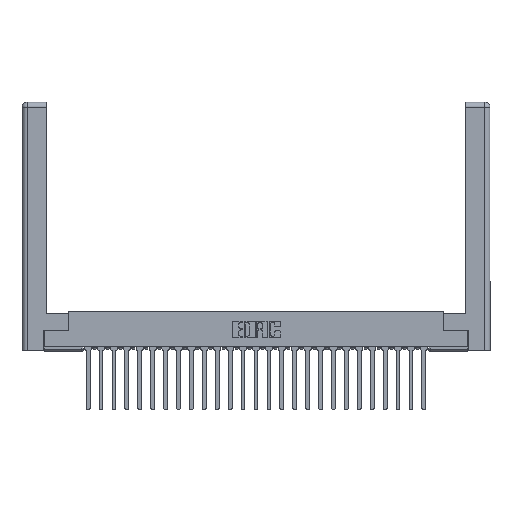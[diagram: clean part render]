
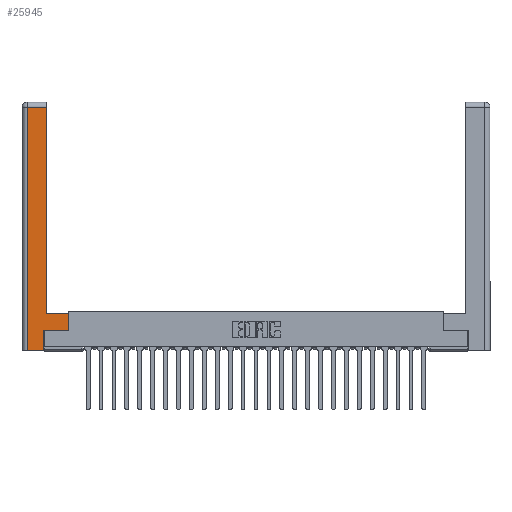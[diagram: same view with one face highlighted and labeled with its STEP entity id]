
A CAD part, top view. The second image highlights one B-rep face of the part: STEP entity #25945.
In plain terms, the highlighted planar face has unit normal (0, 0, 1).
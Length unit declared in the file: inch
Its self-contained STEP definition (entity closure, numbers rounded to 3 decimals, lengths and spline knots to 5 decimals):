
#501 = VECTOR ( 'NONE', #23197, 39.37008 ) ;
#703 = CARTESIAN_POINT ( 'NONE',  ( 0.265, 0., 0. ) ) ;
#752 = CARTESIAN_POINT ( 'NONE',  ( 0.295, 3., 0. ) ) ;
#923 = EDGE_CURVE ( 'NONE', #23110, #20462, #10369, .T. ) ;
#1741 = CARTESIAN_POINT ( 'NONE',  ( 0.265, 0., 0. ) ) ;
#1751 = CARTESIAN_POINT ( 'NONE',  ( 0.0615, 0., 0. ) ) ;
#2740 = LINE ( 'NONE', #17541, #24730 ) ;
#3184 = VECTOR ( 'NONE', #8556, 39.37008 ) ;
#4486 = ORIENTED_EDGE ( 'NONE', *, *, #923, .T. ) ;
#5169 = EDGE_CURVE ( 'NONE', #17542, #25307, #2740, .T. ) ;
#5480 = ORIENTED_EDGE ( 'NONE', *, *, #22704, .T. ) ;
#6525 = LINE ( 'NONE', #6589, #3184 ) ;
#6589 = CARTESIAN_POINT ( 'NONE',  ( 0.565, 0.245, 0. ) ) ;
#6923 = DIRECTION ( 'NONE',  ( 0., 1., 0. ) ) ;
#7065 = CARTESIAN_POINT ( 'NONE',  ( 0.0615, 2.94, 0. ) ) ;
#7544 = VECTOR ( 'NONE', #14274, 39.37008 ) ;
#8556 = DIRECTION ( 'NONE',  ( 1., 0., 0. ) ) ;
#9520 = EDGE_LOOP ( 'NONE', ( #11846, #4486, #5480, #23843, #16336, #23941, #27568, #16644 ) ) ;
#9521 = CARTESIAN_POINT ( 'NONE',  ( 0.295, 2.94, 0. ) ) ;
#9962 = LINE ( 'NONE', #27086, #10650 ) ;
#10175 = DIRECTION ( 'NONE',  ( 0., 0., -1. ) ) ;
#10263 = DIRECTION ( 'NONE',  ( -1., 0., 0. ) ) ;
#10369 = LINE ( 'NONE', #23160, #19050 ) ;
#10650 = VECTOR ( 'NONE', #18647, 39.37008 ) ;
#11282 = VERTEX_POINT ( 'NONE', #23946 ) ;
#11846 = ORIENTED_EDGE ( 'NONE', *, *, #24681, .T. ) ;
#12591 = DIRECTION ( 'NONE',  ( -1., 0., 0. ) ) ;
#13176 = EDGE_CURVE ( 'NONE', #16482, #17907, #6525, .T. ) ;
#14007 = EDGE_CURVE ( 'NONE', #11282, #20609, #21494, .T. ) ;
#14274 = DIRECTION ( 'NONE',  ( 0., 1., 0. ) ) ;
#16336 = ORIENTED_EDGE ( 'NONE', *, *, #25843, .T. ) ;
#16482 = VERTEX_POINT ( 'NONE', #22584 ) ;
#16644 = ORIENTED_EDGE ( 'NONE', *, *, #5169, .T. ) ;
#16682 = PLANE ( 'NONE',  #26206 ) ;
#16854 = LINE ( 'NONE', #1751, #501 ) ;
#16864 = CARTESIAN_POINT ( 'NONE',  ( 0., 0., 0. ) ) ;
#17541 = CARTESIAN_POINT ( 'NONE',  ( 0.295, 0.45, 0. ) ) ;
#17542 = VERTEX_POINT ( 'NONE', #21168 ) ;
#17543 = LINE ( 'NONE', #18364, #7544 ) ;
#17907 = VERTEX_POINT ( 'NONE', #20570 ) ;
#18364 = CARTESIAN_POINT ( 'NONE',  ( 0.265, 0.245, 0. ) ) ;
#18647 = DIRECTION ( 'NONE',  ( 0., 1., 0. ) ) ;
#18700 = DIRECTION ( 'NONE',  ( 1., 0., 0. ) ) ;
#19050 = VECTOR ( 'NONE', #12591, 39.37008 ) ;
#20096 = EDGE_CURVE ( 'NONE', #17907, #17542, #9962, .T. ) ;
#20462 = VERTEX_POINT ( 'NONE', #7065 ) ;
#20570 = CARTESIAN_POINT ( 'NONE',  ( 0.565, 0.245, 0. ) ) ;
#20609 = VERTEX_POINT ( 'NONE', #703 ) ;
#21019 = VECTOR ( 'NONE', #6923, 39.37008 ) ;
#21168 = CARTESIAN_POINT ( 'NONE',  ( 0.565, 0.45, 0. ) ) ;
#21494 = LINE ( 'NONE', #1741, #21834 ) ;
#21659 = LINE ( 'NONE', #752, #21019 ) ;
#21834 = VECTOR ( 'NONE', #18700, 39.37008 ) ;
#21987 = CARTESIAN_POINT ( 'NONE',  ( 0.295, 0.45, 0. ) ) ;
#22245 = FACE_OUTER_BOUND ( 'NONE', #9520, .T. ) ;
#22584 = CARTESIAN_POINT ( 'NONE',  ( 0.265, 0.245, 0. ) ) ;
#22704 = EDGE_CURVE ( 'NONE', #20462, #11282, #16854, .T. ) ;
#23110 = VERTEX_POINT ( 'NONE', #9521 ) ;
#23160 = CARTESIAN_POINT ( 'NONE',  ( 0.0615, 2.94, 0. ) ) ;
#23197 = DIRECTION ( 'NONE',  ( 0., -1., 0. ) ) ;
#23843 = ORIENTED_EDGE ( 'NONE', *, *, #14007, .T. ) ;
#23941 = ORIENTED_EDGE ( 'NONE', *, *, #13176, .T. ) ;
#23946 = CARTESIAN_POINT ( 'NONE',  ( 0.0615, 0., 0. ) ) ;
#24681 = EDGE_CURVE ( 'NONE', #25307, #23110, #21659, .T. ) ;
#24730 = VECTOR ( 'NONE', #26183, 39.37008 ) ;
#25307 = VERTEX_POINT ( 'NONE', #21987 ) ;
#25843 = EDGE_CURVE ( 'NONE', #20609, #16482, #17543, .T. ) ;
#25945 = ADVANCED_FACE ( 'NONE', ( #22245 ), #16682, .F. ) ;
#26183 = DIRECTION ( 'NONE',  ( -1., 0., 0. ) ) ;
#26206 = AXIS2_PLACEMENT_3D ( 'NONE', #16864, #10175, #10263 ) ;
#27086 = CARTESIAN_POINT ( 'NONE',  ( 0.565, 0.45, 0. ) ) ;
#27568 = ORIENTED_EDGE ( 'NONE', *, *, #20096, .T. ) ;
